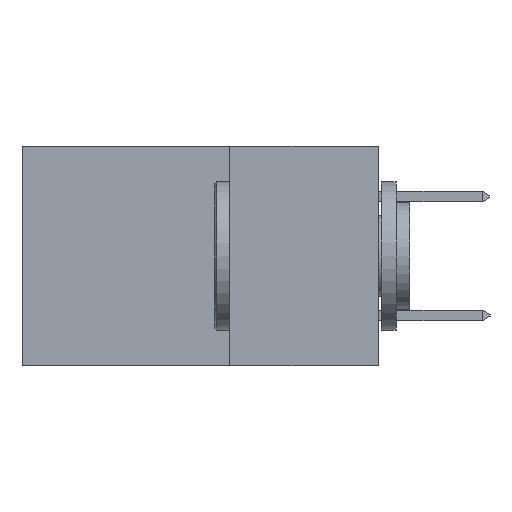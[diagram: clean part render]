
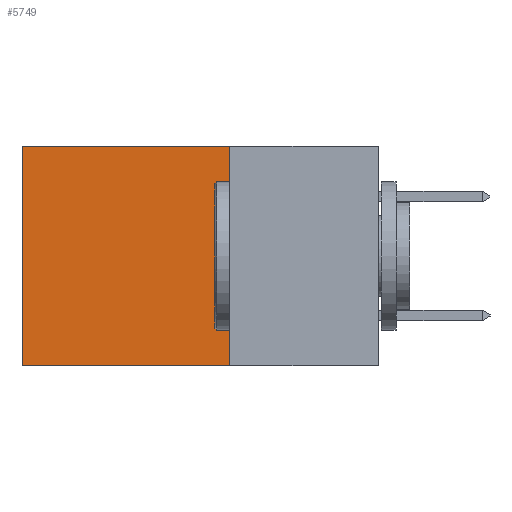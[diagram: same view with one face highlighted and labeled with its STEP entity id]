
A CAD part, left-side view. The second image highlights one B-rep face of the part: STEP entity #5749.
In plain terms, the highlighted planar face has unit normal (-1, 0, 0).
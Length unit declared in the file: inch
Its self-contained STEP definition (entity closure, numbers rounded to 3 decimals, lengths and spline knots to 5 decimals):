
#379 = CARTESIAN_POINT ( 'NONE',  ( 0.2615, 0.6, -0.37 ) ) ;
#540 = DIRECTION ( 'NONE',  ( 0., 1., 0. ) ) ;
#559 = DIRECTION ( 'NONE',  ( 0., 0., -1. ) ) ;
#663 = EDGE_CURVE ( 'NONE', #1893, #9752, #9994, .T. ) ;
#900 = VECTOR ( 'NONE', #540, 39.37008 ) ;
#911 = LINE ( 'NONE', #2420, #2556 ) ;
#1893 = VERTEX_POINT ( 'NONE', #2168 ) ;
#2082 = ORIENTED_EDGE ( 'NONE', *, *, #8582, .F. ) ;
#2168 = CARTESIAN_POINT ( 'NONE',  ( 0.2615, 0.6, 0. ) ) ;
#2420 = CARTESIAN_POINT ( 'NONE',  ( 0.2615, 0.25, -0.37 ) ) ;
#2452 = ORIENTED_EDGE ( 'NONE', *, *, #9017, .T. ) ;
#2556 = VECTOR ( 'NONE', #7261, 39.37008 ) ;
#2851 = VECTOR ( 'NONE', #5477, 39.37008 ) ;
#2902 = EDGE_LOOP ( 'NONE', ( #9933, #6483, #2082, #2452 ) ) ;
#4244 = CARTESIAN_POINT ( 'NONE',  ( 0.2615, 0.25, -0.37 ) ) ;
#4693 = VERTEX_POINT ( 'NONE', #7734 ) ;
#5441 = VERTEX_POINT ( 'NONE', #4244 ) ;
#5477 = DIRECTION ( 'NONE',  ( 0., 1., 0. ) ) ;
#5749 = ADVANCED_FACE ( 'NONE', ( #9511 ), #6096, .F. ) ;
#5917 = DIRECTION ( 'NONE',  ( 0., 0., -1. ) ) ;
#5944 = DIRECTION ( 'NONE',  ( 1., 0., 0. ) ) ;
#6020 = VECTOR ( 'NONE', #559, 39.37008 ) ;
#6025 = CARTESIAN_POINT ( 'NONE',  ( 0.2615, 0.25, -0.37 ) ) ;
#6096 = PLANE ( 'NONE',  #8692 ) ;
#6165 = CARTESIAN_POINT ( 'NONE',  ( 0.2615, 0.25, 0. ) ) ;
#6400 = CARTESIAN_POINT ( 'NONE',  ( 0.2615, 0.6, -0.37 ) ) ;
#6483 = ORIENTED_EDGE ( 'NONE', *, *, #7222, .F. ) ;
#7222 = EDGE_CURVE ( 'NONE', #5441, #9752, #9245, .T. ) ;
#7261 = DIRECTION ( 'NONE',  ( 0., 0., -1. ) ) ;
#7734 = CARTESIAN_POINT ( 'NONE',  ( 0.2615, 0.25, 0. ) ) ;
#7908 = CARTESIAN_POINT ( 'NONE',  ( 0.2615, 0.25, -0.37 ) ) ;
#8582 = EDGE_CURVE ( 'NONE', #4693, #5441, #911, .T. ) ;
#8692 = AXIS2_PLACEMENT_3D ( 'NONE', #6025, #5944, #5917 ) ;
#9017 = EDGE_CURVE ( 'NONE', #4693, #1893, #9447, .T. ) ;
#9245 = LINE ( 'NONE', #7908, #2851 ) ;
#9447 = LINE ( 'NONE', #6165, #900 ) ;
#9511 = FACE_OUTER_BOUND ( 'NONE', #2902, .T. ) ;
#9752 = VERTEX_POINT ( 'NONE', #6400 ) ;
#9933 = ORIENTED_EDGE ( 'NONE', *, *, #663, .T. ) ;
#9994 = LINE ( 'NONE', #379, #6020 ) ;
